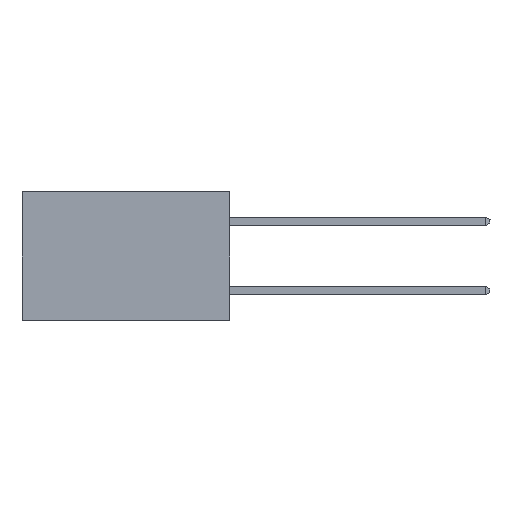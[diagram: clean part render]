
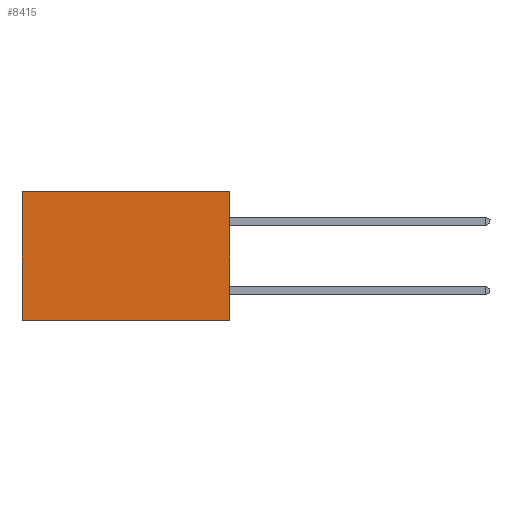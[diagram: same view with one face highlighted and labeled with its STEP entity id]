
A CAD part, left-side view. The second image highlights one B-rep face of the part: STEP entity #8415.
In plain terms, the highlighted planar face has unit normal (-1, 0, 0).
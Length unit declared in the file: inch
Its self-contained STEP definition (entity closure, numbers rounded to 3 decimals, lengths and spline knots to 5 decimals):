
#23 = ORIENTED_EDGE ( 'NONE', *, *, #2613, .F. ) ;
#157 = PLANE ( 'NONE',  #11120 ) ;
#647 = ORIENTED_EDGE ( 'NONE', *, *, #6230, .T. ) ;
#915 = VERTEX_POINT ( 'NONE', #7498 ) ;
#991 = VERTEX_POINT ( 'NONE', #6571 ) ;
#1097 = DIRECTION ( 'NONE',  ( 0., 0., -1. ) ) ;
#2122 = VECTOR ( 'NONE', #10224, 39.37008 ) ;
#2507 = ORIENTED_EDGE ( 'NONE', *, *, #8312, .F. ) ;
#2613 = EDGE_CURVE ( 'NONE', #915, #991, #9381, .T. ) ;
#3373 = LINE ( 'NONE', #4454, #2122 ) ;
#3472 = CARTESIAN_POINT ( 'NONE',  ( 0.2615, 0.6, -0.37 ) ) ;
#4045 = DIRECTION ( 'NONE',  ( 1., 0., 0. ) ) ;
#4454 = CARTESIAN_POINT ( 'NONE',  ( 0.2615, 0.6, -0.37 ) ) ;
#4566 = DIRECTION ( 'NONE',  ( 0., 1., 0. ) ) ;
#4641 = VERTEX_POINT ( 'NONE', #11540 ) ;
#4883 = VERTEX_POINT ( 'NONE', #3472 ) ;
#6230 = EDGE_CURVE ( 'NONE', #4641, #4883, #3373, .T. ) ;
#6309 = DIRECTION ( 'NONE',  ( 0., 0., -1. ) ) ;
#6571 = CARTESIAN_POINT ( 'NONE',  ( 0.2615, 0., -0.37 ) ) ;
#7310 = VECTOR ( 'NONE', #7882, 39.37008 ) ;
#7498 = CARTESIAN_POINT ( 'NONE',  ( 0.2615, 0., 0. ) ) ;
#7823 = CARTESIAN_POINT ( 'NONE',  ( 0.2615, 0., -0.37 ) ) ;
#7882 = DIRECTION ( 'NONE',  ( 0., 1., 0. ) ) ;
#8107 = EDGE_CURVE ( 'NONE', #915, #4641, #10271, .T. ) ;
#8312 = EDGE_CURVE ( 'NONE', #991, #4883, #9018, .T. ) ;
#8415 = ADVANCED_FACE ( 'NONE', ( #11642 ), #157, .F. ) ;
#8451 = CARTESIAN_POINT ( 'NONE',  ( 0.2615, 0., -0.37 ) ) ;
#9018 = LINE ( 'NONE', #7823, #7310 ) ;
#9381 = LINE ( 'NONE', #8451, #9805 ) ;
#9805 = VECTOR ( 'NONE', #6309, 39.37008 ) ;
#10142 = CARTESIAN_POINT ( 'NONE',  ( 0.2615, 0., 0. ) ) ;
#10224 = DIRECTION ( 'NONE',  ( 0., 0., -1. ) ) ;
#10271 = LINE ( 'NONE', #10142, #11111 ) ;
#10752 = EDGE_LOOP ( 'NONE', ( #647, #2507, #23, #11339 ) ) ;
#10888 = CARTESIAN_POINT ( 'NONE',  ( 0.2615, 0., -0.37 ) ) ;
#11111 = VECTOR ( 'NONE', #4566, 39.37008 ) ;
#11120 = AXIS2_PLACEMENT_3D ( 'NONE', #10888, #4045, #1097 ) ;
#11339 = ORIENTED_EDGE ( 'NONE', *, *, #8107, .T. ) ;
#11540 = CARTESIAN_POINT ( 'NONE',  ( 0.2615, 0.6, 0. ) ) ;
#11642 = FACE_OUTER_BOUND ( 'NONE', #10752, .T. ) ;
